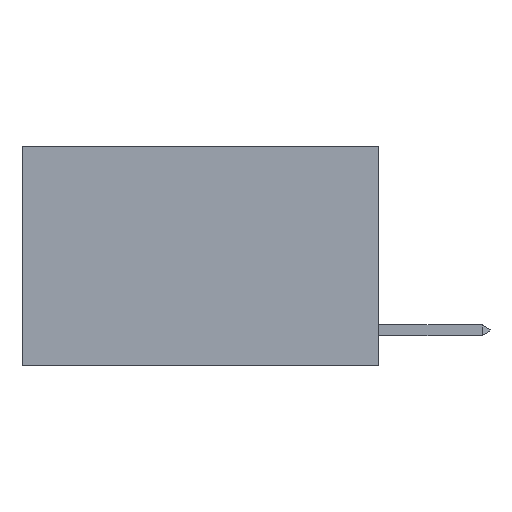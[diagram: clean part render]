
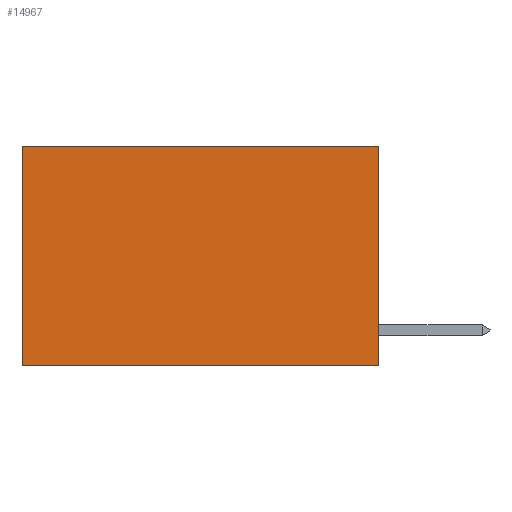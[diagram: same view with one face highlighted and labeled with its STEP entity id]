
A CAD part, left-side view. The second image highlights one B-rep face of the part: STEP entity #14967.
In plain terms, the highlighted planar face has unit normal (-1, 0, 0).
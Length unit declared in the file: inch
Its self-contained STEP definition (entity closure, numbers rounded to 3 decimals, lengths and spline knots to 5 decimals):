
#136 = CARTESIAN_POINT ( 'NONE',  ( 0.2625, 0.6, 0. ) ) ;
#1407 = EDGE_CURVE ( 'NONE', #7573, #10918, #3622, .T. ) ;
#1962 = DIRECTION ( 'NONE',  ( 0., 1., 0. ) ) ;
#2278 = CARTESIAN_POINT ( 'NONE',  ( 0.2625, 0., 0. ) ) ;
#2517 = EDGE_CURVE ( 'NONE', #17754, #7573, #14621, .T. ) ;
#3112 = CARTESIAN_POINT ( 'NONE',  ( 0.2625, 0., 0. ) ) ;
#3622 = LINE ( 'NONE', #136, #7428 ) ;
#4004 = VECTOR ( 'NONE', #15384, 39.37008 ) ;
#4768 = DIRECTION ( 'NONE',  ( 0., 0., -1. ) ) ;
#4793 = VECTOR ( 'NONE', #1962, 39.37008 ) ;
#6173 = DIRECTION ( 'NONE',  ( 0., 1., 0. ) ) ;
#7428 = VECTOR ( 'NONE', #18013, 39.37008 ) ;
#7573 = VERTEX_POINT ( 'NONE', #11658 ) ;
#7714 = CARTESIAN_POINT ( 'NONE',  ( 0.2625, 0., -0.37 ) ) ;
#7980 = VERTEX_POINT ( 'NONE', #7714 ) ;
#8296 = LINE ( 'NONE', #10441, #4004 ) ;
#10441 = CARTESIAN_POINT ( 'NONE',  ( 0.2625, 0., 0. ) ) ;
#10627 = FACE_OUTER_BOUND ( 'NONE', #10751, .T. ) ;
#10751 = EDGE_LOOP ( 'NONE', ( #19460, #20668, #14401, #16698 ) ) ;
#10918 = VERTEX_POINT ( 'NONE', #11775 ) ;
#11658 = CARTESIAN_POINT ( 'NONE',  ( 0.2625, 0.6, 0. ) ) ;
#11740 = CARTESIAN_POINT ( 'NONE',  ( 0.2625, 0., -0.37 ) ) ;
#11775 = CARTESIAN_POINT ( 'NONE',  ( 0.2625, 0.6, -0.37 ) ) ;
#12949 = LINE ( 'NONE', #11740, #4793 ) ;
#14401 = ORIENTED_EDGE ( 'NONE', *, *, #15335, .F. ) ;
#14546 = DIRECTION ( 'NONE',  ( 1., 0., 0. ) ) ;
#14621 = LINE ( 'NONE', #20793, #16813 ) ;
#14641 = EDGE_CURVE ( 'NONE', #7980, #10918, #12949, .T. ) ;
#14967 = ADVANCED_FACE ( 'NONE', ( #10627 ), #16105, .F. ) ;
#15335 = EDGE_CURVE ( 'NONE', #17754, #7980, #8296, .T. ) ;
#15384 = DIRECTION ( 'NONE',  ( 0., 0., -1. ) ) ;
#16105 = PLANE ( 'NONE',  #18909 ) ;
#16698 = ORIENTED_EDGE ( 'NONE', *, *, #2517, .T. ) ;
#16813 = VECTOR ( 'NONE', #6173, 39.37008 ) ;
#17754 = VERTEX_POINT ( 'NONE', #2278 ) ;
#18013 = DIRECTION ( 'NONE',  ( 0., 0., -1. ) ) ;
#18909 = AXIS2_PLACEMENT_3D ( 'NONE', #3112, #14546, #4768 ) ;
#19460 = ORIENTED_EDGE ( 'NONE', *, *, #1407, .T. ) ;
#20668 = ORIENTED_EDGE ( 'NONE', *, *, #14641, .F. ) ;
#20793 = CARTESIAN_POINT ( 'NONE',  ( 0.2625, 0., 0. ) ) ;
